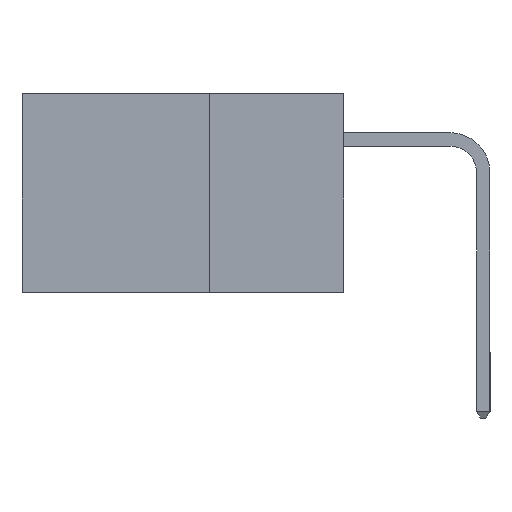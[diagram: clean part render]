
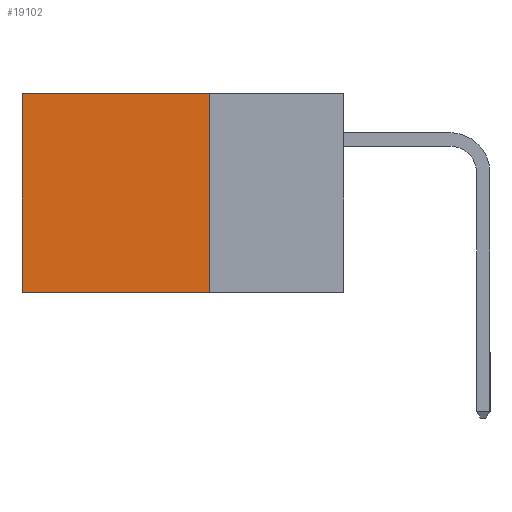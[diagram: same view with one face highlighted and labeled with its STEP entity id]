
A CAD part, left-side view. The second image highlights one B-rep face of the part: STEP entity #19102.
In plain terms, the highlighted planar face has unit normal (-1, 0, 0).
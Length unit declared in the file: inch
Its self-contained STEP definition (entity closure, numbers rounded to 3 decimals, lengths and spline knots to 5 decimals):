
#434 = DIRECTION ( 'NONE',  ( 0., 0., -1. ) ) ;
#446 = ORIENTED_EDGE ( 'NONE', *, *, #18335, .F. ) ;
#527 = ORIENTED_EDGE ( 'NONE', *, *, #13766, .T. ) ;
#1099 = CARTESIAN_POINT ( 'NONE',  ( 0.298, 0.25, 0. ) ) ;
#1277 = DIRECTION ( 'NONE',  ( 0., 0., -1. ) ) ;
#1850 = CARTESIAN_POINT ( 'NONE',  ( 0.298, 0.25, 0. ) ) ;
#3380 = ORIENTED_EDGE ( 'NONE', *, *, #16043, .T. ) ;
#4365 = VECTOR ( 'NONE', #434, 39.37008 ) ;
#4701 = DIRECTION ( 'NONE',  ( 0., 1., 0. ) ) ;
#5680 = DIRECTION ( 'NONE',  ( 0., 1., 0. ) ) ;
#6321 = LINE ( 'NONE', #21998, #4365 ) ;
#8333 = EDGE_CURVE ( 'NONE', #24227, #21152, #23538, .T. ) ;
#9144 = DIRECTION ( 'NONE',  ( 1., 0., 0. ) ) ;
#10733 = VECTOR ( 'NONE', #5680, 39.37008 ) ;
#10787 = CARTESIAN_POINT ( 'NONE',  ( 0.298, 0.25, -0.37 ) ) ;
#13766 = EDGE_CURVE ( 'NONE', #15993, #17983, #16159, .T. ) ;
#13946 = CARTESIAN_POINT ( 'NONE',  ( 0.298, 0.25, 0. ) ) ;
#15714 = DIRECTION ( 'NONE',  ( 0., 0., -1. ) ) ;
#15993 = VERTEX_POINT ( 'NONE', #1850 ) ;
#16043 = EDGE_CURVE ( 'NONE', #17983, #21152, #6321, .T. ) ;
#16159 = LINE ( 'NONE', #22243, #10733 ) ;
#17596 = EDGE_LOOP ( 'NONE', ( #3380, #24305, #446, #527 ) ) ;
#17983 = VERTEX_POINT ( 'NONE', #19182 ) ;
#18335 = EDGE_CURVE ( 'NONE', #15993, #24227, #23098, .T. ) ;
#19102 = ADVANCED_FACE ( 'NONE', ( #23372 ), #25605, .F. ) ;
#19182 = CARTESIAN_POINT ( 'NONE',  ( 0.298, 0.6, 0. ) ) ;
#19275 = VECTOR ( 'NONE', #15714, 39.37008 ) ;
#21152 = VERTEX_POINT ( 'NONE', #25729 ) ;
#21998 = CARTESIAN_POINT ( 'NONE',  ( 0.298, 0.6, 0. ) ) ;
#22243 = CARTESIAN_POINT ( 'NONE',  ( 0.298, 0.25, 0. ) ) ;
#22613 = VECTOR ( 'NONE', #4701, 39.37008 ) ;
#23098 = LINE ( 'NONE', #13946, #19275 ) ;
#23372 = FACE_OUTER_BOUND ( 'NONE', #17596, .T. ) ;
#23538 = LINE ( 'NONE', #10787, #22613 ) ;
#24227 = VERTEX_POINT ( 'NONE', #25334 ) ;
#24305 = ORIENTED_EDGE ( 'NONE', *, *, #8333, .F. ) ;
#25334 = CARTESIAN_POINT ( 'NONE',  ( 0.298, 0.25, -0.37 ) ) ;
#25605 = PLANE ( 'NONE',  #25828 ) ;
#25729 = CARTESIAN_POINT ( 'NONE',  ( 0.298, 0.6, -0.37 ) ) ;
#25828 = AXIS2_PLACEMENT_3D ( 'NONE', #1099, #9144, #1277 ) ;
